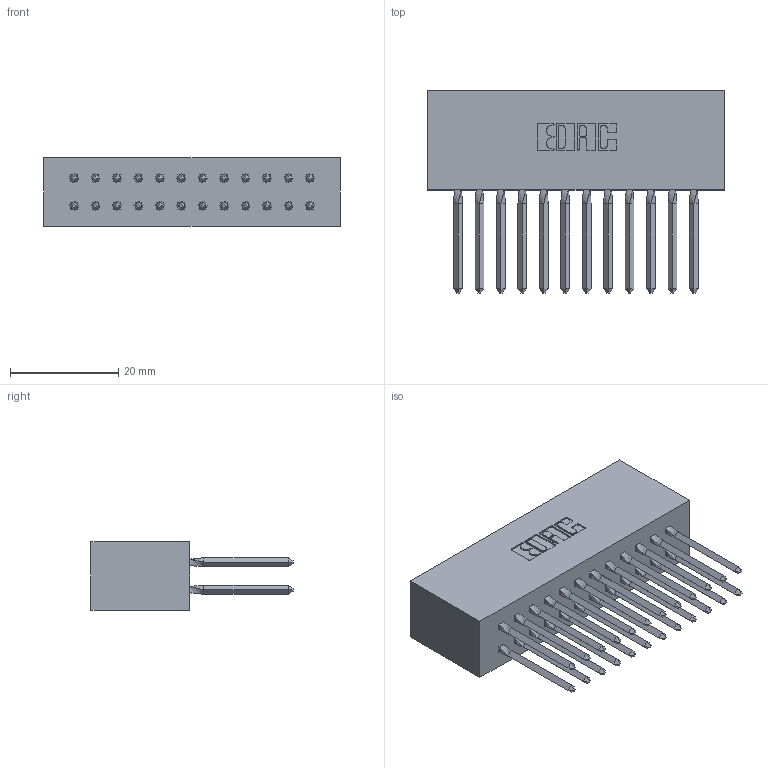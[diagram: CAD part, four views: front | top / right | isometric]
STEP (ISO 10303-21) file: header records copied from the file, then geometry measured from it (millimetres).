
FILE_DESCRIPTION (( 'STEP AP203' ), '1' );
FILE_NAME ('317-024-542-801.STEP', '2020-02-27T18:09:29', ( '' ), ( '' ), 'SwSTEP 2.0', 'SolidWorks 2016', '' );
FILE_SCHEMA (( 'CONFIG_CONTROL_DESIGN' ));
Length unit declared in the file: inch
Products named in the file (3): 317-290-003_542; 317 Part_Lugless; 317-024-542-801
Assembly tree (25 placements, depth 2):
  317-024-542-801
    317 Part_Lugless
    317-290-003_542  x24
Bounding box: 54.76 x 37.34 x 12.7 mm (x, y, z)
Volume: 9749.4 mm3; surface area: 12771.5 mm2
Topology: 25 solids, 25 shells, 1458 faces, 4079 edges, 2606 vertices
Faces by surface type: plane 1154, cylinder 208, bspline 96
Entity records: 20139 total; most frequent: CARTESIAN_POINT 3757, ORIENTED_EDGE 3420, DIRECTION 2922, EDGE_CURVE 1710, VECTOR 1548, LINE 1548, VERTEX_POINT 1134, AXIS2_PLACEMENT_3D 687
